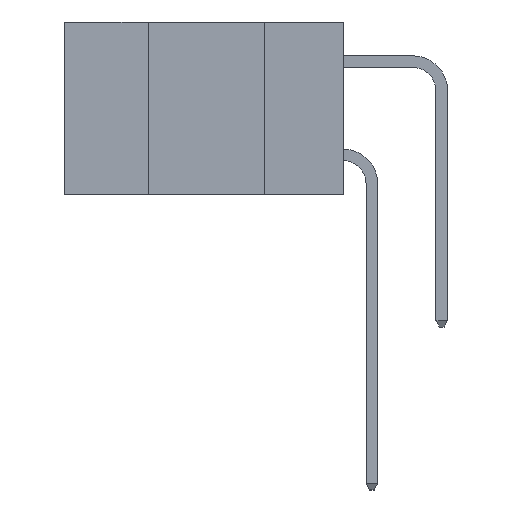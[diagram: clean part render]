
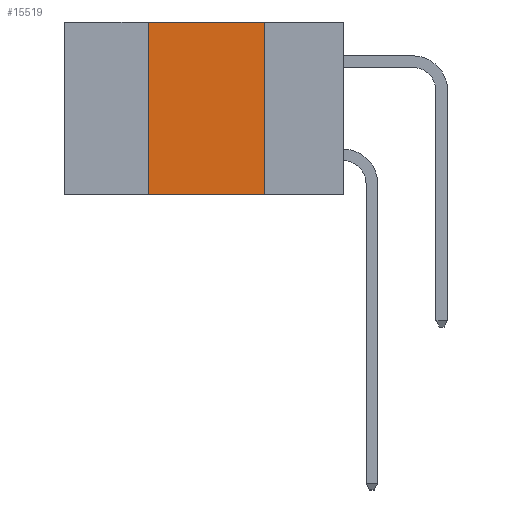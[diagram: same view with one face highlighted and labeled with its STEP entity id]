
A CAD part, left-side view. The second image highlights one B-rep face of the part: STEP entity #15519.
In plain terms, the highlighted planar face has unit normal (-1, 0, 0).
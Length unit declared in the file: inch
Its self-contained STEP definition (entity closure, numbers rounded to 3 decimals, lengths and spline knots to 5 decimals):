
#139 = EDGE_LOOP ( 'NONE', ( #12663, #4879, #7254, #12851 ) ) ;
#1052 = DIRECTION ( 'NONE',  ( 0., -1., 0. ) ) ;
#1561 = VECTOR ( 'NONE', #11572, 39.37008 ) ;
#2344 = EDGE_CURVE ( 'NONE', #17639, #2971, #17107, .T. ) ;
#2971 = VERTEX_POINT ( 'NONE', #7068 ) ;
#3755 = DIRECTION ( 'NONE',  ( 1., 0., 0. ) ) ;
#4879 = ORIENTED_EDGE ( 'NONE', *, *, #17209, .F. ) ;
#4899 = LINE ( 'NONE', #11555, #1561 ) ;
#6347 = VERTEX_POINT ( 'NONE', #11883 ) ;
#6404 = VECTOR ( 'NONE', #1052, 39.37008 ) ;
#7068 = CARTESIAN_POINT ( 'NONE',  ( 0., 0.17, -0.37 ) ) ;
#7254 = ORIENTED_EDGE ( 'NONE', *, *, #13755, .F. ) ;
#8042 = CARTESIAN_POINT ( 'NONE',  ( 0., 0.42, -0.37 ) ) ;
#8208 = CARTESIAN_POINT ( 'NONE',  ( 0., 0.17, -0.37 ) ) ;
#8234 = VECTOR ( 'NONE', #17343, 39.37008 ) ;
#8532 = AXIS2_PLACEMENT_3D ( 'NONE', #17195, #3755, #13363 ) ;
#9245 = EDGE_CURVE ( 'NONE', #12359, #2971, #4899, .T. ) ;
#9284 = PLANE ( 'NONE',  #8532 ) ;
#9320 = DIRECTION ( 'NONE',  ( 0., 0., -1. ) ) ;
#10412 = FACE_OUTER_BOUND ( 'NONE', #139, .T. ) ;
#10889 = CARTESIAN_POINT ( 'NONE',  ( 0., 0.6, 0. ) ) ;
#11555 = CARTESIAN_POINT ( 'NONE',  ( 0., 0.6, -0.37 ) ) ;
#11572 = DIRECTION ( 'NONE',  ( 0., -1., 0. ) ) ;
#11770 = CARTESIAN_POINT ( 'NONE',  ( 0., 0.17, 0. ) ) ;
#11877 = CARTESIAN_POINT ( 'NONE',  ( 0., 0.42, -0.37 ) ) ;
#11883 = CARTESIAN_POINT ( 'NONE',  ( 0., 0.42, 0. ) ) ;
#12359 = VERTEX_POINT ( 'NONE', #11877 ) ;
#12663 = ORIENTED_EDGE ( 'NONE', *, *, #2344, .F. ) ;
#12851 = ORIENTED_EDGE ( 'NONE', *, *, #9245, .T. ) ;
#13363 = DIRECTION ( 'NONE',  ( 0., 0., -1. ) ) ;
#13649 = LINE ( 'NONE', #10889, #6404 ) ;
#13755 = EDGE_CURVE ( 'NONE', #12359, #6347, #15013, .T. ) ;
#15013 = LINE ( 'NONE', #8042, #8234 ) ;
#15519 = ADVANCED_FACE ( 'NONE', ( #10412 ), #9284, .F. ) ;
#16734 = VECTOR ( 'NONE', #9320, 39.37008 ) ;
#17107 = LINE ( 'NONE', #8208, #16734 ) ;
#17195 = CARTESIAN_POINT ( 'NONE',  ( 0., 0.6, 0. ) ) ;
#17209 = EDGE_CURVE ( 'NONE', #6347, #17639, #13649, .T. ) ;
#17343 = DIRECTION ( 'NONE',  ( 0., 0., 1. ) ) ;
#17639 = VERTEX_POINT ( 'NONE', #11770 ) ;
